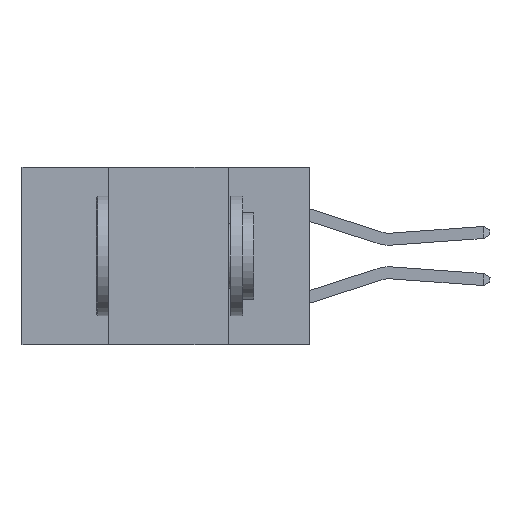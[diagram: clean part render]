
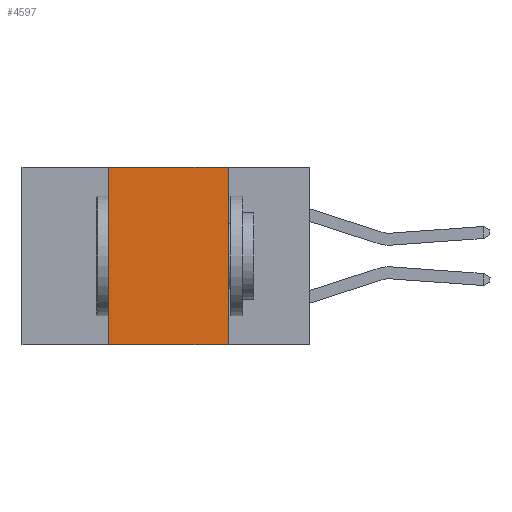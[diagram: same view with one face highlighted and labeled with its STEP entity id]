
A CAD part, left-side view. The second image highlights one B-rep face of the part: STEP entity #4597.
In plain terms, the highlighted planar face has unit normal (-1, 0, 0).
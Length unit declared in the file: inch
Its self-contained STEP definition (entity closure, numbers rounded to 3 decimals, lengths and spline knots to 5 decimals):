
#235 = LINE ( 'NONE', #282, #5333 ) ;
#248 = EDGE_CURVE ( 'NONE', #8591, #5141, #4283, .T. ) ;
#282 = CARTESIAN_POINT ( 'NONE',  ( 0., 0.6, 0. ) ) ;
#1415 = CARTESIAN_POINT ( 'NONE',  ( 0., 0.6, 0. ) ) ;
#1435 = DIRECTION ( 'NONE',  ( 0., -1., 0. ) ) ;
#1982 = CARTESIAN_POINT ( 'NONE',  ( 0., 0.17, 0. ) ) ;
#2150 = AXIS2_PLACEMENT_3D ( 'NONE', #1415, #7057, #5171 ) ;
#2152 = ORIENTED_EDGE ( 'NONE', *, *, #248, .T. ) ;
#2297 = EDGE_CURVE ( 'NONE', #8591, #6570, #6009, .T. ) ;
#2969 = ORIENTED_EDGE ( 'NONE', *, *, #10123, .F. ) ;
#3201 = CARTESIAN_POINT ( 'NONE',  ( 0., 0.17, 0. ) ) ;
#3342 = LINE ( 'NONE', #3201, #10112 ) ;
#3707 = EDGE_LOOP ( 'NONE', ( #2969, #5115, #8315, #2152 ) ) ;
#3874 = CARTESIAN_POINT ( 'NONE',  ( 0., 0.17, -0.37 ) ) ;
#4283 = LINE ( 'NONE', #7971, #6487 ) ;
#4597 = ADVANCED_FACE ( 'NONE', ( #11863 ), #8827, .F. ) ;
#4839 = DIRECTION ( 'NONE',  ( 0., -1., 0. ) ) ;
#5115 = ORIENTED_EDGE ( 'NONE', *, *, #6805, .F. ) ;
#5141 = VERTEX_POINT ( 'NONE', #3874 ) ;
#5171 = DIRECTION ( 'NONE',  ( 0., 0., -1. ) ) ;
#5333 = VECTOR ( 'NONE', #4839, 39.37008 ) ;
#5424 = CARTESIAN_POINT ( 'NONE',  ( 0., 0.42, 0. ) ) ;
#5546 = VECTOR ( 'NONE', #7237, 39.37008 ) ;
#5855 = VERTEX_POINT ( 'NONE', #1982 ) ;
#6009 = LINE ( 'NONE', #5424, #5546 ) ;
#6487 = VECTOR ( 'NONE', #1435, 39.37008 ) ;
#6570 = VERTEX_POINT ( 'NONE', #10952 ) ;
#6805 = EDGE_CURVE ( 'NONE', #6570, #5855, #235, .T. ) ;
#7057 = DIRECTION ( 'NONE',  ( 1., 0., 0. ) ) ;
#7237 = DIRECTION ( 'NONE',  ( 0., 0., 1. ) ) ;
#7971 = CARTESIAN_POINT ( 'NONE',  ( 0., 0.6, -0.37 ) ) ;
#8315 = ORIENTED_EDGE ( 'NONE', *, *, #2297, .F. ) ;
#8591 = VERTEX_POINT ( 'NONE', #11506 ) ;
#8827 = PLANE ( 'NONE',  #2150 ) ;
#9823 = DIRECTION ( 'NONE',  ( 0., 0., -1. ) ) ;
#10112 = VECTOR ( 'NONE', #9823, 39.37008 ) ;
#10123 = EDGE_CURVE ( 'NONE', #5855, #5141, #3342, .T. ) ;
#10952 = CARTESIAN_POINT ( 'NONE',  ( 0., 0.42, 0. ) ) ;
#11506 = CARTESIAN_POINT ( 'NONE',  ( 0., 0.42, -0.37 ) ) ;
#11863 = FACE_OUTER_BOUND ( 'NONE', #3707, .T. ) ;
